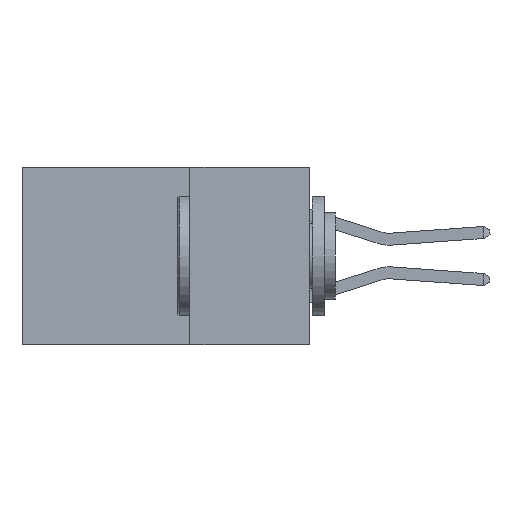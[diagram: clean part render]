
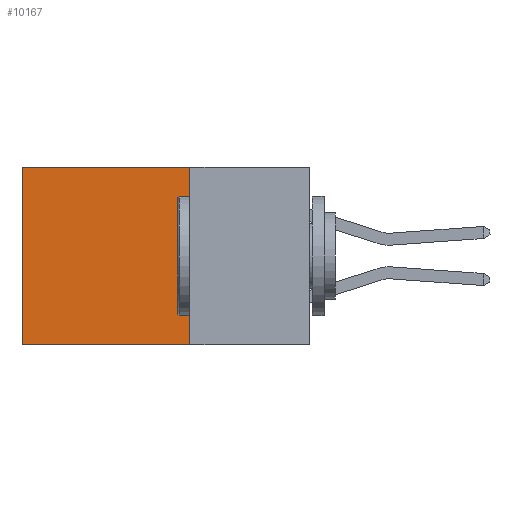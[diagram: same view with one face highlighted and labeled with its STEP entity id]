
A CAD part, left-side view. The second image highlights one B-rep face of the part: STEP entity #10167.
In plain terms, the highlighted planar face has unit normal (-1, 0, 0).
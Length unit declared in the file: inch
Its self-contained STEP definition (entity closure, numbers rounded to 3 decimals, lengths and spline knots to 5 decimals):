
#234 = EDGE_CURVE ( 'NONE', #12274, #4512, #15558, .T. ) ;
#332 = PLANE ( 'NONE',  #12643 ) ;
#372 = CARTESIAN_POINT ( 'NONE',  ( 0.298, 0.25, 0. ) ) ;
#1875 = DIRECTION ( 'NONE',  ( 0., 0., -1. ) ) ;
#1896 = LINE ( 'NONE', #6867, #10993 ) ;
#2045 = VERTEX_POINT ( 'NONE', #8478 ) ;
#2200 = VECTOR ( 'NONE', #1875, 39.37008 ) ;
#2532 = CARTESIAN_POINT ( 'NONE',  ( 0.298, 0.25, -0.37 ) ) ;
#2880 = CARTESIAN_POINT ( 'NONE',  ( 0.298, 0.25, 0. ) ) ;
#3811 = DIRECTION ( 'NONE',  ( 0., 1., 0. ) ) ;
#4512 = VERTEX_POINT ( 'NONE', #14119 ) ;
#4927 = VERTEX_POINT ( 'NONE', #7832 ) ;
#5496 = ORIENTED_EDGE ( 'NONE', *, *, #8897, .T. ) ;
#5795 = CARTESIAN_POINT ( 'NONE',  ( 0.298, 0.25, -0.37 ) ) ;
#5803 = VECTOR ( 'NONE', #13861, 39.37008 ) ;
#5889 = VECTOR ( 'NONE', #3811, 39.37008 ) ;
#5915 = LINE ( 'NONE', #10563, #2200 ) ;
#6619 = DIRECTION ( 'NONE',  ( 1., 0., 0. ) ) ;
#6740 = DIRECTION ( 'NONE',  ( 0., 0., -1. ) ) ;
#6827 = EDGE_CURVE ( 'NONE', #4927, #12274, #1896, .T. ) ;
#6867 = CARTESIAN_POINT ( 'NONE',  ( 0.298, 0.25, 0. ) ) ;
#7832 = CARTESIAN_POINT ( 'NONE',  ( 0.298, 0.25, 0. ) ) ;
#8196 = EDGE_LOOP ( 'NONE', ( #5496, #9346, #12615, #10572 ) ) ;
#8478 = CARTESIAN_POINT ( 'NONE',  ( 0.298, 0.6, 0. ) ) ;
#8897 = EDGE_CURVE ( 'NONE', #2045, #4512, #5915, .T. ) ;
#9346 = ORIENTED_EDGE ( 'NONE', *, *, #234, .F. ) ;
#10167 = ADVANCED_FACE ( 'NONE', ( #13529 ), #332, .F. ) ;
#10563 = CARTESIAN_POINT ( 'NONE',  ( 0.298, 0.6, 0. ) ) ;
#10572 = ORIENTED_EDGE ( 'NONE', *, *, #14246, .T. ) ;
#10993 = VECTOR ( 'NONE', #6740, 39.37008 ) ;
#12274 = VERTEX_POINT ( 'NONE', #5795 ) ;
#12615 = ORIENTED_EDGE ( 'NONE', *, *, #6827, .F. ) ;
#12643 = AXIS2_PLACEMENT_3D ( 'NONE', #2880, #6619, #15113 ) ;
#13529 = FACE_OUTER_BOUND ( 'NONE', #8196, .T. ) ;
#13861 = DIRECTION ( 'NONE',  ( 0., 1., 0. ) ) ;
#14119 = CARTESIAN_POINT ( 'NONE',  ( 0.298, 0.6, -0.37 ) ) ;
#14246 = EDGE_CURVE ( 'NONE', #4927, #2045, #15480, .T. ) ;
#15113 = DIRECTION ( 'NONE',  ( 0., 0., -1. ) ) ;
#15480 = LINE ( 'NONE', #372, #5803 ) ;
#15558 = LINE ( 'NONE', #2532, #5889 ) ;
